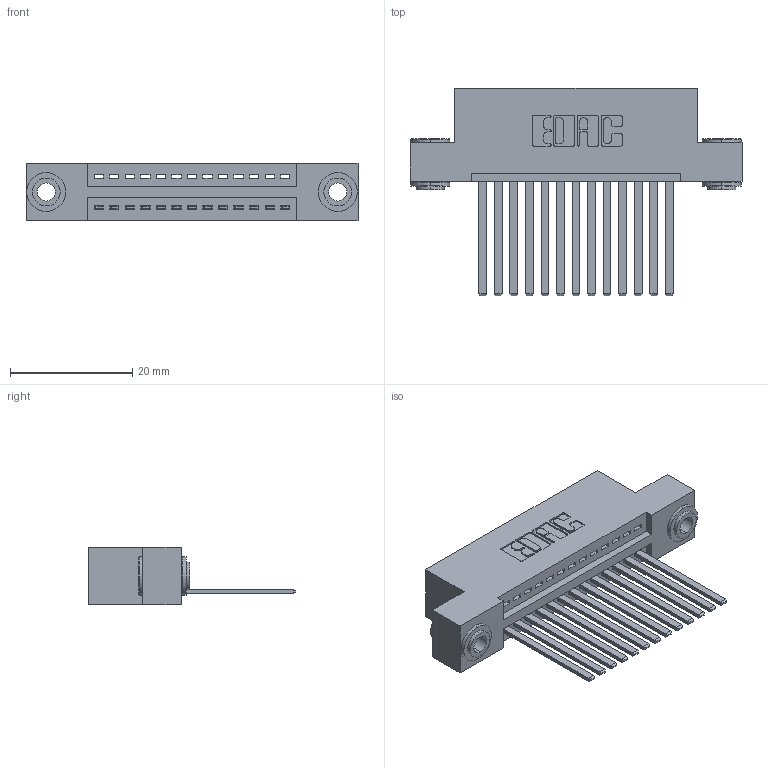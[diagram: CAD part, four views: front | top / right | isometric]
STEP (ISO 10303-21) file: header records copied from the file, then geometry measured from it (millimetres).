
FILE_DESCRIPTION (( 'STEP AP203' ), '1' );
FILE_NAME ('395-013-544-103.STEP', '2018-11-05T21:33:05', ( '' ), ( '' ), 'SwSTEP 2.0', 'SolidWorks 2016', '' );
FILE_SCHEMA (( 'CONFIG_CONTROL_DESIGN' ));
Length unit declared in the file: inch
Products named in the file (4): 395-013-544-103; 345-292-001_345-293-144; 345 Part_Flush Mounting Lugs - 0.156 Dia-TH; 345-250-002_345-250-002-102
Assembly tree (16 placements, depth 2):
  395-013-544-103
    345 Part_Flush Mounting Lugs - 0.156 Dia-TH
    345-292-001_345-293-144  x13
    345-250-002_345-250-002-102  x2
Bounding box: 54.23 x 33.96 x 9.4 mm (x, y, z)
Volume: 5083.1 mm3; surface area: 7027.3 mm2
Topology: 16 solids, 16 shells, 840 faces, 2471 edges, 1626 vertices
Faces by surface type: plane 558, cylinder 274, cone 8
Entity records: 14154 total; most frequent: CARTESIAN_POINT 2430, ORIENTED_EDGE 2370, DIRECTION 2193, EDGE_CURVE 1185, VECTOR 981, LINE 981, VERTEX_POINT 786, AXIS2_PLACEMENT_3D 606
